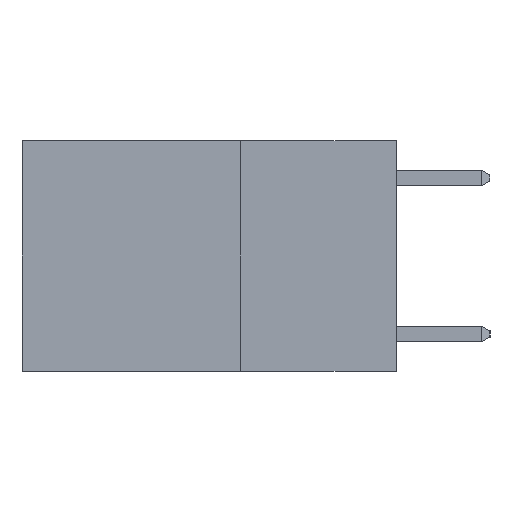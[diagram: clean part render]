
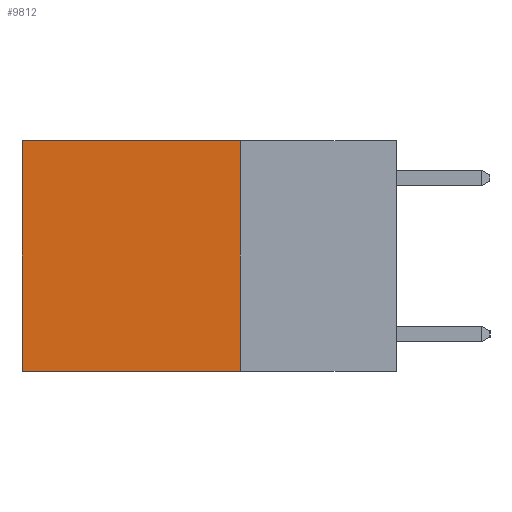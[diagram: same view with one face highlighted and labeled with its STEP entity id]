
A CAD part, left-side view. The second image highlights one B-rep face of the part: STEP entity #9812.
In plain terms, the highlighted planar face has unit normal (-1, 0, 0).
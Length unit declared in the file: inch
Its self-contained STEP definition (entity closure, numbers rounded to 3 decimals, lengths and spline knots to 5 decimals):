
#18 = FACE_OUTER_BOUND ( 'NONE', #3961, .T. ) ;
#440 = ORIENTED_EDGE ( 'NONE', *, *, #7302, .F. ) ;
#471 = CARTESIAN_POINT ( 'NONE',  ( 0.2625, 0.6, 0. ) ) ;
#1092 = DIRECTION ( 'NONE',  ( 0., 0., -1. ) ) ;
#1266 = DIRECTION ( 'NONE',  ( 0., 0., -1. ) ) ;
#1267 = EDGE_CURVE ( 'NONE', #2987, #2262, #6585, .T. ) ;
#2059 = CARTESIAN_POINT ( 'NONE',  ( 0.2625, 0.25, -0.37 ) ) ;
#2239 = CARTESIAN_POINT ( 'NONE',  ( 0.2625, 0.25, -0.37 ) ) ;
#2262 = VERTEX_POINT ( 'NONE', #3984 ) ;
#2600 = VECTOR ( 'NONE', #8837, 39.37008 ) ;
#2638 = PLANE ( 'NONE',  #4634 ) ;
#2987 = VERTEX_POINT ( 'NONE', #8198 ) ;
#3417 = DIRECTION ( 'NONE',  ( 1., 0., 0. ) ) ;
#3961 = EDGE_LOOP ( 'NONE', ( #8672, #6252, #440, #8978 ) ) ;
#3984 = CARTESIAN_POINT ( 'NONE',  ( 0.2625, 0.6, 0. ) ) ;
#4312 = DIRECTION ( 'NONE',  ( 0., 1., 0. ) ) ;
#4321 = CARTESIAN_POINT ( 'NONE',  ( 0.2625, 0.25, 0. ) ) ;
#4634 = AXIS2_PLACEMENT_3D ( 'NONE', #4891, #3417, #8657 ) ;
#4891 = CARTESIAN_POINT ( 'NONE',  ( 0.2625, 0.25, 0. ) ) ;
#5073 = VECTOR ( 'NONE', #4312, 39.37008 ) ;
#5251 = VERTEX_POINT ( 'NONE', #6532 ) ;
#6226 = LINE ( 'NONE', #471, #7993 ) ;
#6252 = ORIENTED_EDGE ( 'NONE', *, *, #7490, .F. ) ;
#6378 = CARTESIAN_POINT ( 'NONE',  ( 0.2625, 0.25, 0. ) ) ;
#6532 = CARTESIAN_POINT ( 'NONE',  ( 0.2625, 0.6, -0.37 ) ) ;
#6585 = LINE ( 'NONE', #4321, #5073 ) ;
#6595 = LINE ( 'NONE', #2059, #2600 ) ;
#6723 = VECTOR ( 'NONE', #1092, 39.37008 ) ;
#6961 = VERTEX_POINT ( 'NONE', #2239 ) ;
#7302 = EDGE_CURVE ( 'NONE', #2987, #6961, #8484, .T. ) ;
#7490 = EDGE_CURVE ( 'NONE', #6961, #5251, #6595, .T. ) ;
#7993 = VECTOR ( 'NONE', #1266, 39.37008 ) ;
#8198 = CARTESIAN_POINT ( 'NONE',  ( 0.2625, 0.25, 0. ) ) ;
#8484 = LINE ( 'NONE', #6378, #6723 ) ;
#8614 = EDGE_CURVE ( 'NONE', #2262, #5251, #6226, .T. ) ;
#8657 = DIRECTION ( 'NONE',  ( 0., 0., -1. ) ) ;
#8672 = ORIENTED_EDGE ( 'NONE', *, *, #8614, .T. ) ;
#8837 = DIRECTION ( 'NONE',  ( 0., 1., 0. ) ) ;
#8978 = ORIENTED_EDGE ( 'NONE', *, *, #1267, .T. ) ;
#9812 = ADVANCED_FACE ( 'NONE', ( #18 ), #2638, .F. ) ;
